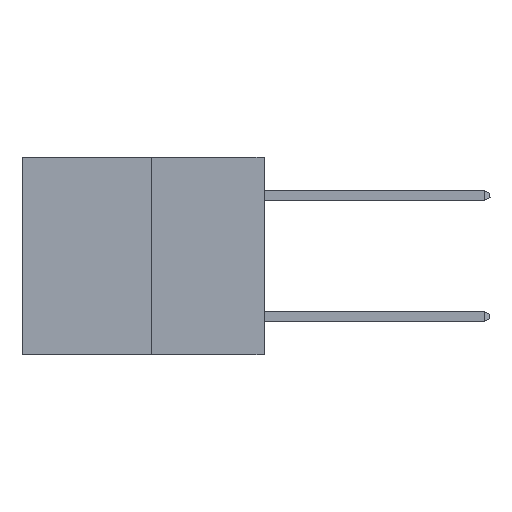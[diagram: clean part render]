
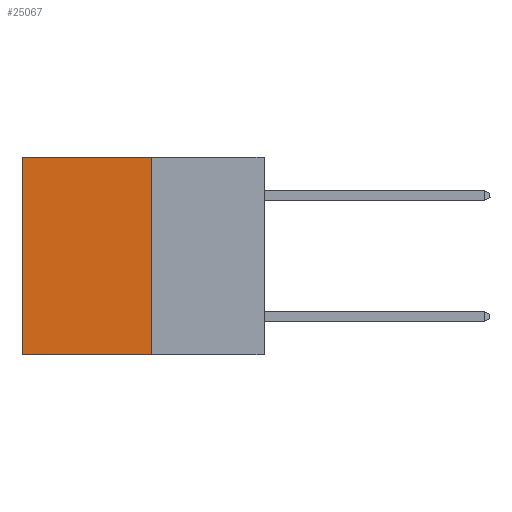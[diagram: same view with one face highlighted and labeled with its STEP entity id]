
A CAD part, left-side view. The second image highlights one B-rep face of the part: STEP entity #25067.
In plain terms, the highlighted planar face has unit normal (-1, 0, 0).
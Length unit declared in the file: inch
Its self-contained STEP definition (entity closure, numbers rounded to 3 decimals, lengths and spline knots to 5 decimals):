
#318 = CARTESIAN_POINT ( 'NONE',  ( 0.3165, 0.6, -0.49 ) ) ;
#405 = EDGE_LOOP ( 'NONE', ( #16162, #13136, #1515, #24959 ) ) ;
#1515 = ORIENTED_EDGE ( 'NONE', *, *, #19340, .F. ) ;
#1549 = EDGE_CURVE ( 'NONE', #22464, #4616, #6710, .T. ) ;
#1726 = CARTESIAN_POINT ( 'NONE',  ( 0.3165, 0.28, -0.49 ) ) ;
#1823 = CARTESIAN_POINT ( 'NONE',  ( 0.3165, 0.6, -0.49 ) ) ;
#1995 = DIRECTION ( 'NONE',  ( 0., 0., -1. ) ) ;
#4616 = VERTEX_POINT ( 'NONE', #26281 ) ;
#5706 = AXIS2_PLACEMENT_3D ( 'NONE', #6697, #23637, #21397 ) ;
#6049 = LINE ( 'NONE', #14275, #23586 ) ;
#6697 = CARTESIAN_POINT ( 'NONE',  ( 0.3165, 0.28, -0.49 ) ) ;
#6710 = LINE ( 'NONE', #11668, #14693 ) ;
#7392 = VERTEX_POINT ( 'NONE', #1823 ) ;
#8166 = VECTOR ( 'NONE', #1995, 39.37008 ) ;
#10190 = LINE ( 'NONE', #318, #20112 ) ;
#11668 = CARTESIAN_POINT ( 'NONE',  ( 0.3165, 0.28, 0. ) ) ;
#13136 = ORIENTED_EDGE ( 'NONE', *, *, #21698, .F. ) ;
#14199 = VERTEX_POINT ( 'NONE', #1726 ) ;
#14275 = CARTESIAN_POINT ( 'NONE',  ( 0.3165, 0.28, -0.49 ) ) ;
#14354 = DIRECTION ( 'NONE',  ( 0., 1., 0. ) ) ;
#14693 = VECTOR ( 'NONE', #14354, 39.37008 ) ;
#14834 = FACE_OUTER_BOUND ( 'NONE', #405, .T. ) ;
#16162 = ORIENTED_EDGE ( 'NONE', *, *, #18344, .T. ) ;
#17286 = PLANE ( 'NONE',  #5706 ) ;
#18344 = EDGE_CURVE ( 'NONE', #4616, #7392, #10190, .T. ) ;
#19340 = EDGE_CURVE ( 'NONE', #22464, #14199, #22743, .T. ) ;
#20112 = VECTOR ( 'NONE', #27168, 39.37008 ) ;
#21397 = DIRECTION ( 'NONE',  ( 0., 0., -1. ) ) ;
#21698 = EDGE_CURVE ( 'NONE', #14199, #7392, #6049, .T. ) ;
#22464 = VERTEX_POINT ( 'NONE', #22813 ) ;
#22482 = DIRECTION ( 'NONE',  ( 0., 1., 0. ) ) ;
#22743 = LINE ( 'NONE', #27137, #8166 ) ;
#22813 = CARTESIAN_POINT ( 'NONE',  ( 0.3165, 0.28, 0. ) ) ;
#23586 = VECTOR ( 'NONE', #22482, 39.37008 ) ;
#23637 = DIRECTION ( 'NONE',  ( 1., 0., 0. ) ) ;
#24959 = ORIENTED_EDGE ( 'NONE', *, *, #1549, .T. ) ;
#25067 = ADVANCED_FACE ( 'NONE', ( #14834 ), #17286, .F. ) ;
#26281 = CARTESIAN_POINT ( 'NONE',  ( 0.3165, 0.6, 0. ) ) ;
#27137 = CARTESIAN_POINT ( 'NONE',  ( 0.3165, 0.28, -0.49 ) ) ;
#27168 = DIRECTION ( 'NONE',  ( 0., 0., -1. ) ) ;
